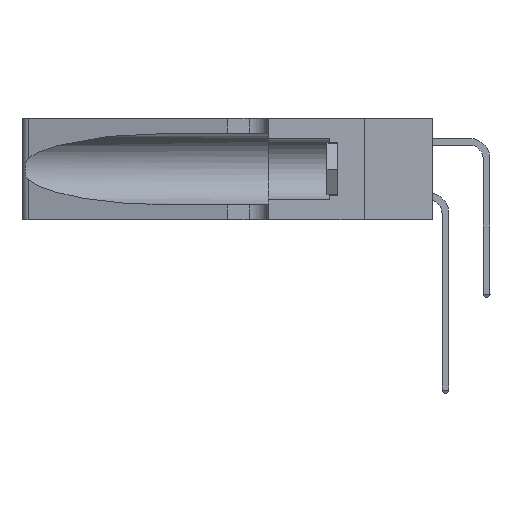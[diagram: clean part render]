
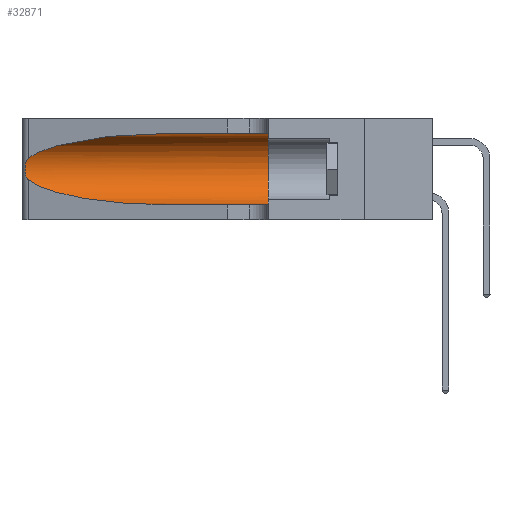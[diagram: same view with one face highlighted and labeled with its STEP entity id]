
A CAD part, left-side view. The second image highlights one B-rep face of the part: STEP entity #32871.
In plain terms, the highlighted cylindrical face has radius 3.308 mm (diameter 6.617 mm), a partial arc.
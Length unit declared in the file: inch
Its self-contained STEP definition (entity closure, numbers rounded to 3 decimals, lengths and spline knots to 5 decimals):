
#461 =( BOUNDED_CURVE ( )  B_SPLINE_CURVE ( 3, ( #26484, #13352, #29138, #13459 ),
 .UNSPECIFIED., .F., .F. ) 
 B_SPLINE_CURVE_WITH_KNOTS ( ( 4, 4 ),
 ( 1.5708, 2.84003 ),
 .UNSPECIFIED. ) 
 CURVE ( )  GEOMETRIC_REPRESENTATION_ITEM ( )  RATIONAL_B_SPLINE_CURVE ( ( 1., 0.87, 0.87, 1. ) ) 
 REPRESENTATION_ITEM ( '' )  );
#897 = CARTESIAN_POINT ( 'NONE',  ( 0.1305, 0.72297, 0.05475 ) ) ;
#1025 = CARTESIAN_POINT ( 'NONE',  ( 0.25555, 1.22993, 0.14849 ) ) ;
#1138 = CARTESIAN_POINT ( 'NONE',  ( 0.25487, 1.22718, 0.22369 ) ) ;
#1283 = AXIS2_PLACEMENT_3D ( 'NONE', #30939, #12680, #12471 ) ;
#2744 = EDGE_CURVE ( 'NONE', #12097, #6267, #20993, .T. ) ;
#3285 = CARTESIAN_POINT ( 'NONE',  ( 0.2373, 1.15595, 0.08982 ) ) ;
#3520 = CARTESIAN_POINT ( 'NONE',  ( 0.25787, 1.23484, 0.2124 ) ) ;
#4472 = CARTESIAN_POINT ( 'NONE',  ( 0.1305, 0.72297, 0.31525 ) ) ;
#5289 = CARTESIAN_POINT ( 'NONE',  ( 0.25487, 1.22718, 0.22369 ) ) ;
#5569 = ORIENTED_EDGE ( 'NONE', *, *, #23924, .T. ) ;
#5803 = VECTOR ( 'NONE', #23536, 39.37008 ) ;
#6007 = VERTEX_POINT ( 'NONE', #6037 ) ;
#6037 = CARTESIAN_POINT ( 'NONE',  ( 0.1305, 0.72297, 0.05475 ) ) ;
#6267 = VERTEX_POINT ( 'NONE', #31894 ) ;
#6269 = CARTESIAN_POINT ( 'NONE',  ( 0.25487, 1.22718, 0.14631 ) ) ;
#6320 = EDGE_LOOP ( 'NONE', ( #15937, #5569, #24202, #27196, #12294, #31202 ) ) ;
#6815 = EDGE_CURVE ( 'NONE', #8281, #6007, #32088, .T. ) ;
#7769 = VERTEX_POINT ( 'NONE', #4472 ) ;
#8190 = DIRECTION ( 'NONE',  ( 0., -1., 0. ) ) ;
#8281 = VERTEX_POINT ( 'NONE', #32820 ) ;
#8537 = LINE ( 'NONE', #8809, #18263 ) ;
#8809 = CARTESIAN_POINT ( 'NONE',  ( 0.1305, 1.61858, 0.31525 ) ) ;
#10465 = AXIS2_PLACEMENT_3D ( 'NONE', #29081, #8190, #15895 ) ;
#11341 = CARTESIAN_POINT ( 'NONE',  ( 0.25789, 1.23486, 0.15765 ) ) ;
#12097 = VERTEX_POINT ( 'NONE', #25973 ) ;
#12294 = ORIENTED_EDGE ( 'NONE', *, *, #2744, .F. ) ;
#12471 = DIRECTION ( 'NONE',  ( 0., 0., 1. ) ) ;
#12680 = DIRECTION ( 'NONE',  ( 0., 1., 0. ) ) ;
#13328 = CARTESIAN_POINT ( 'NONE',  ( 0.1305, 1.61858, 0.05475 ) ) ;
#13352 = CARTESIAN_POINT ( 'NONE',  ( 0.18966, 0.96281, 0.31525 ) ) ;
#13459 = CARTESIAN_POINT ( 'NONE',  ( 0.25487, 1.22718, 0.22369 ) ) ;
#13947 = CARTESIAN_POINT ( 'NONE',  ( 0.26075, 1.23896, 0.19203 ) ) ;
#14071 = EDGE_CURVE ( 'NONE', #7769, #12097, #8537, .T. ) ;
#14302 = CARTESIAN_POINT ( 'NONE',  ( 0.26075, 1.23896, 0.178 ) ) ;
#14981 = VERTEX_POINT ( 'NONE', #5289 ) ;
#15148 = LINE ( 'NONE', #13328, #5803 ) ;
#15895 = DIRECTION ( 'NONE',  ( 0., 0., -1. ) ) ;
#15937 = ORIENTED_EDGE ( 'NONE', *, *, #22082, .T. ) ;
#16551 = CARTESIAN_POINT ( 'NONE',  ( 0.25639, 1.23186, 0.15144 ) ) ;
#16746 = DIRECTION ( 'NONE',  ( 0., -1., 0. ) ) ;
#17861 = CYLINDRICAL_SURFACE ( 'NONE', #10465, 0.13025 ) ;
#18263 = VECTOR ( 'NONE', #16746, 39.37008 ) ;
#19014 = CARTESIAN_POINT ( 'NONE',  ( 0.25639, 1.23184, 0.21858 ) ) ;
#20993 = CIRCLE ( 'NONE', #1283, 0.13025 ) ;
#21108 = FACE_OUTER_BOUND ( 'NONE', #6320, .T. ) ;
#22082 = EDGE_CURVE ( 'NONE', #7769, #14981, #461, .T. ) ;
#22109 = CARTESIAN_POINT ( 'NONE',  ( 0.26017, 1.23833, 0.17102 ) ) ;
#23536 = DIRECTION ( 'NONE',  ( 0., -1., 0. ) ) ;
#23924 = EDGE_CURVE ( 'NONE', #14981, #8281, #31672, .T. ) ;
#24202 = ORIENTED_EDGE ( 'NONE', *, *, #6815, .T. ) ;
#24350 = CARTESIAN_POINT ( 'NONE',  ( 0.26018, 1.23835, 0.19895 ) ) ;
#25973 = CARTESIAN_POINT ( 'NONE',  ( 0.1305, 0.35, 0.31525 ) ) ;
#26279 = CARTESIAN_POINT ( 'NONE',  ( 0.25487, 1.22718, 0.14631 ) ) ;
#26347 = EDGE_CURVE ( 'NONE', #6007, #6267, #15148, .T. ) ;
#26484 = CARTESIAN_POINT ( 'NONE',  ( 0.1305, 0.72297, 0.31525 ) ) ;
#26727 = CARTESIAN_POINT ( 'NONE',  ( 0.18966, 0.96281, 0.05475 ) ) ;
#27196 = ORIENTED_EDGE ( 'NONE', *, *, #26347, .T. ) ;
#27204 = CARTESIAN_POINT ( 'NONE',  ( 0.25555, 1.22994, 0.2215 ) ) ;
#29081 = CARTESIAN_POINT ( 'NONE',  ( 0.1305, 1.61858, 0.185 ) ) ;
#29138 = CARTESIAN_POINT ( 'NONE',  ( 0.2373, 1.15595, 0.28018 ) ) ;
#29624 = CARTESIAN_POINT ( 'NONE',  ( 0.25854, 1.2359, 0.20912 ) ) ;
#30939 = CARTESIAN_POINT ( 'NONE',  ( 0.1305, 0.35, 0.185 ) ) ;
#31202 = ORIENTED_EDGE ( 'NONE', *, *, #14071, .F. ) ;
#31672 = B_SPLINE_CURVE_WITH_KNOTS ( 'NONE', 3,
 ( #1138, #27204, #19014, #3520, #29624, #24350, #13947, #14302, #22109, #32076, #11341, #16551, #1025, #6269 ),
 .UNSPECIFIED., .F., .F.,
 ( 4, 2, 2, 2, 2, 2, 4 ),
 ( 0., 0.00027, 0.00053, 0.00107, 0.0016, 0.00187, 0.00214 ),
 .UNSPECIFIED. ) ;
#31894 = CARTESIAN_POINT ( 'NONE',  ( 0.1305, 0.35, 0.05475 ) ) ;
#32076 = CARTESIAN_POINT ( 'NONE',  ( 0.25856, 1.23593, 0.16098 ) ) ;
#32088 =( BOUNDED_CURVE ( )  B_SPLINE_CURVE ( 3, ( #26279, #3285, #26727, #897 ),
 .UNSPECIFIED., .F., .T. ) 
 B_SPLINE_CURVE_WITH_KNOTS ( ( 4, 4 ),
 ( 3.44316, 4.71239 ),
 .UNSPECIFIED. ) 
 CURVE ( )  GEOMETRIC_REPRESENTATION_ITEM ( )  RATIONAL_B_SPLINE_CURVE ( ( 1., 0.87, 0.87, 1. ) ) 
 REPRESENTATION_ITEM ( '' )  );
#32820 = CARTESIAN_POINT ( 'NONE',  ( 0.25487, 1.22718, 0.14631 ) ) ;
#32871 = ADVANCED_FACE ( 'NONE', ( #21108 ), #17861, .F. ) ;
